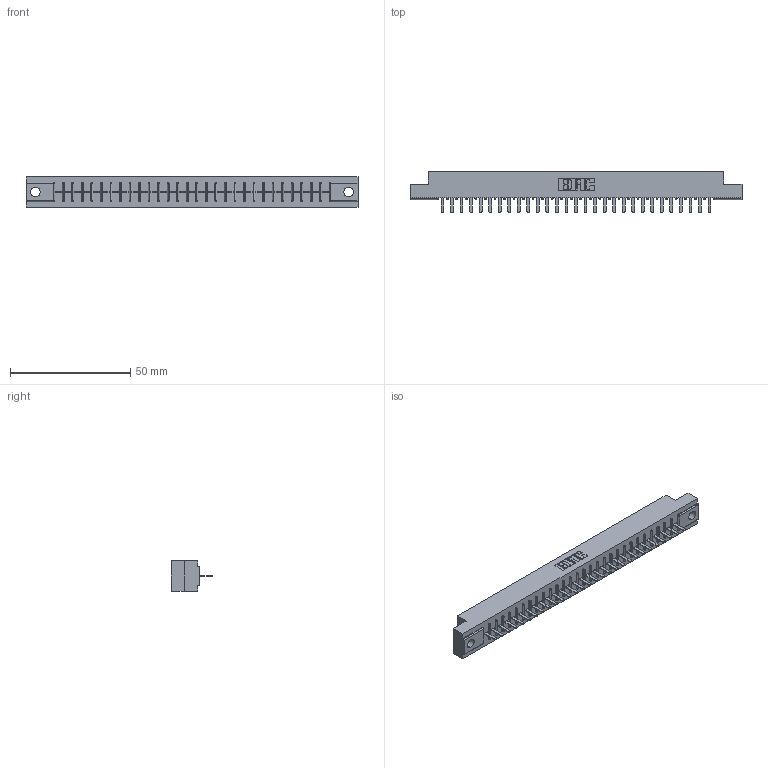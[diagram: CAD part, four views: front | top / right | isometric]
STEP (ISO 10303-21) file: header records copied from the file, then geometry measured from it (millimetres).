
FILE_DESCRIPTION (( 'STEP AP203' ), '1' );
FILE_NAME ('356-029-420-104.STEP', '2020-09-23T19:00:13', ( '' ), ( '' ), 'SwSTEP 2.0', 'SolidWorks 2020', '' );
FILE_SCHEMA (( 'CONFIG_CONTROL_DESIGN' ));
Length unit declared in the file: inch
Products named in the file (3): 306-290-001_120; 356-029-420-104; 306 Part_.156 Dia
Assembly tree (30 placements, depth 2):
  356-029-420-104
    306 Part_.156 Dia
    306-290-001_120  x29
Bounding box: 137.92 x 17.12 x 12.7 mm (x, y, z)
Volume: 15029.1 mm3; surface area: 15118.8 mm2
Topology: 30 solids, 30 shells, 2160 faces, 6065 edges, 3886 vertices
Faces by surface type: plane 1445, cylinder 599, sphere 116
Entity records: 29102 total; most frequent: CARTESIAN_POINT 4888, ORIENTED_EDGE 4842, DIRECTION 4813, EDGE_CURVE 2421, VECTOR 1895, LINE 1895, VERTEX_POINT 1534, AXIS2_PLACEMENT_3D 1459
